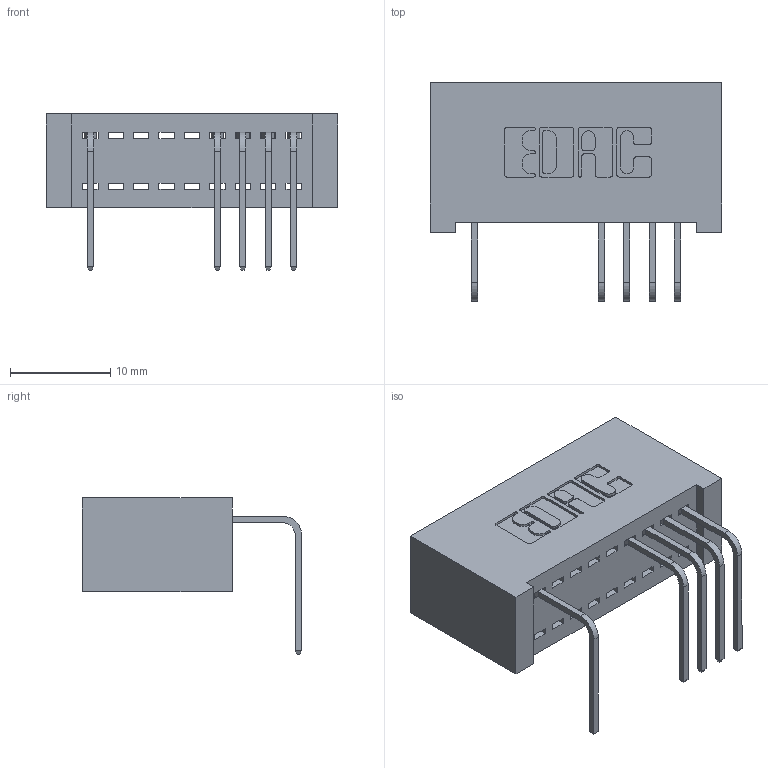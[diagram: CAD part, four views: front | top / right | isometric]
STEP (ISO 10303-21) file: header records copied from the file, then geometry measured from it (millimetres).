
FILE_DESCRIPTION (( 'STEP AP203' ), '1' );
FILE_NAME ('342-009-558-101.STEP', '2018-08-10T12:59:27', ( '' ), ( '' ), 'SwSTEP 2.0', 'SolidWorks 2016', '' );
FILE_SCHEMA (( 'CONFIG_CONTROL_DESIGN' ));
Length unit declared in the file: inch
Products named in the file (3): 342 Part_Lugless; 345-292-001_558 Tail - 2; 342-009-558-101
Assembly tree (6 placements, depth 2):
  342-009-558-101
    342 Part_Lugless
    345-292-001_558 Tail - 2  x5
Bounding box: 29.11 x 21.91 x 15.62 mm (x, y, z)
Volume: 2810.6 mm3; surface area: 3691.9 mm2
Topology: 6 solids, 6 shells, 450 faces, 1353 edges, 894 vertices
Faces by surface type: plane 330, cylinder 120
Entity records: 9317 total; most frequent: CARTESIAN_POINT 1637, ORIENTED_EDGE 1586, DIRECTION 1435, EDGE_CURVE 793, LINE 673, VECTOR 673, VERTEX_POINT 526, AXIS2_PLACEMENT_3D 381
